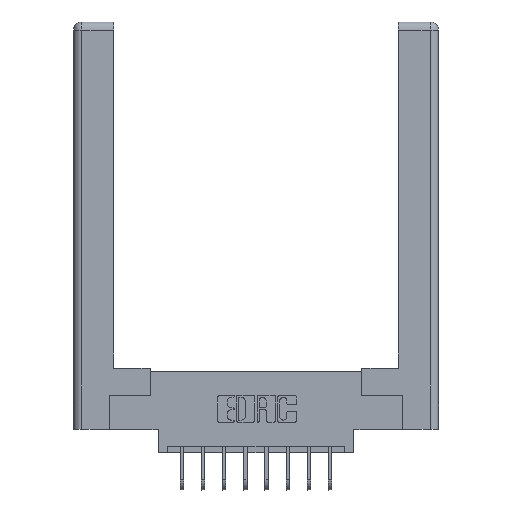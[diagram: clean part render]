
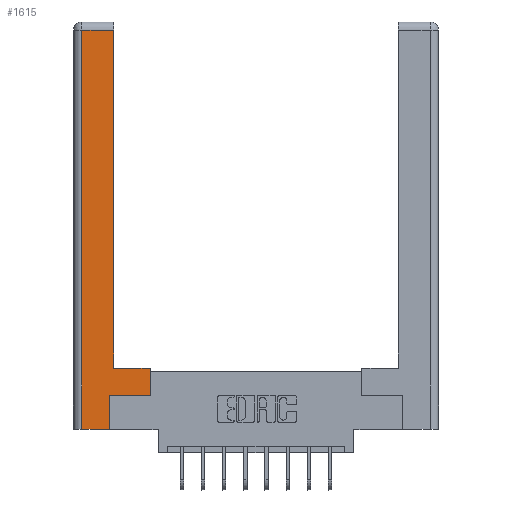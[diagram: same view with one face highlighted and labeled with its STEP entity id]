
A CAD part, top view. The second image highlights one B-rep face of the part: STEP entity #1615.
In plain terms, the highlighted planar face has unit normal (0, 0, 1).
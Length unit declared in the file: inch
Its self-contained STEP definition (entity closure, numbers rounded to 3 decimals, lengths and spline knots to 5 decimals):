
#156 = CARTESIAN_POINT ( 'NONE',  ( 0.265, 0.245, 0. ) ) ;
#361 = ORIENTED_EDGE ( 'NONE', *, *, #6981, .T. ) ;
#690 = CARTESIAN_POINT ( 'NONE',  ( 0.0615, 0., 0. ) ) ;
#691 = CARTESIAN_POINT ( 'NONE',  ( 0.565, 0.245, 0. ) ) ;
#766 = VECTOR ( 'NONE', #13962, 39.37008 ) ;
#854 = ORIENTED_EDGE ( 'NONE', *, *, #11714, .T. ) ;
#1370 = ORIENTED_EDGE ( 'NONE', *, *, #6584, .T. ) ;
#1501 = EDGE_CURVE ( 'NONE', #4162, #12065, #8631, .T. ) ;
#1615 = ADVANCED_FACE ( 'NONE', ( #4391 ), #9600, .F. ) ;
#1638 = VECTOR ( 'NONE', #10856, 39.37008 ) ;
#1649 = VECTOR ( 'NONE', #15169, 39.37008 ) ;
#2095 = VERTEX_POINT ( 'NONE', #2620 ) ;
#2319 = EDGE_CURVE ( 'NONE', #12065, #2095, #7311, .T. ) ;
#2481 = CARTESIAN_POINT ( 'NONE',  ( 0., 0., 0. ) ) ;
#2620 = CARTESIAN_POINT ( 'NONE',  ( 0.295, 0.45, 0. ) ) ;
#2752 = EDGE_CURVE ( 'NONE', #12931, #4162, #7843, .T. ) ;
#3084 = DIRECTION ( 'NONE',  ( 0., 1., 0. ) ) ;
#3595 = DIRECTION ( 'NONE',  ( 0., -1., 0. ) ) ;
#3642 = DIRECTION ( 'NONE',  ( 0., 0., -1. ) ) ;
#3760 = LINE ( 'NONE', #7287, #11484 ) ;
#3936 = AXIS2_PLACEMENT_3D ( 'NONE', #2481, #3642, #4826 ) ;
#4162 = VERTEX_POINT ( 'NONE', #691 ) ;
#4369 = CARTESIAN_POINT ( 'NONE',  ( 0.265, 0., 0. ) ) ;
#4391 = FACE_OUTER_BOUND ( 'NONE', #10382, .T. ) ;
#4430 = LINE ( 'NONE', #11430, #14558 ) ;
#4826 = DIRECTION ( 'NONE',  ( -1., 0., 0. ) ) ;
#4856 = EDGE_CURVE ( 'NONE', #7955, #14331, #3760, .T. ) ;
#5141 = ORIENTED_EDGE ( 'NONE', *, *, #1501, .T. ) ;
#5241 = DIRECTION ( 'NONE',  ( -1., 0., 0. ) ) ;
#5264 = VECTOR ( 'NONE', #7913, 39.37008 ) ;
#5302 = VERTEX_POINT ( 'NONE', #4369 ) ;
#5493 = CARTESIAN_POINT ( 'NONE',  ( 0.265, 0.245, 0. ) ) ;
#5680 = CARTESIAN_POINT ( 'NONE',  ( 0.295, 3., 0. ) ) ;
#5685 = LINE ( 'NONE', #5680, #766 ) ;
#5876 = EDGE_CURVE ( 'NONE', #5302, #12931, #7757, .T. ) ;
#6104 = ORIENTED_EDGE ( 'NONE', *, *, #2752, .T. ) ;
#6584 = EDGE_CURVE ( 'NONE', #14049, #7955, #7743, .T. ) ;
#6746 = CARTESIAN_POINT ( 'NONE',  ( 0.565, 0.245, 0. ) ) ;
#6981 = EDGE_CURVE ( 'NONE', #2095, #14049, #5685, .T. ) ;
#7035 = VECTOR ( 'NONE', #3084, 39.37008 ) ;
#7287 = CARTESIAN_POINT ( 'NONE',  ( 0.0615, 0., 0. ) ) ;
#7311 = LINE ( 'NONE', #11934, #1638 ) ;
#7551 = VECTOR ( 'NONE', #5241, 39.37008 ) ;
#7743 = LINE ( 'NONE', #13588, #7551 ) ;
#7757 = LINE ( 'NONE', #156, #7035 ) ;
#7843 = LINE ( 'NONE', #6746, #5264 ) ;
#7913 = DIRECTION ( 'NONE',  ( 1., 0., 0. ) ) ;
#7955 = VERTEX_POINT ( 'NONE', #13560 ) ;
#8631 = LINE ( 'NONE', #13912, #1649 ) ;
#8905 = CARTESIAN_POINT ( 'NONE',  ( 0.565, 0.45, 0. ) ) ;
#9097 = ORIENTED_EDGE ( 'NONE', *, *, #5876, .T. ) ;
#9600 = PLANE ( 'NONE',  #3936 ) ;
#10382 = EDGE_LOOP ( 'NONE', ( #361, #1370, #12322, #854, #9097, #6104, #5141, #11536 ) ) ;
#10856 = DIRECTION ( 'NONE',  ( -1., 0., 0. ) ) ;
#11373 = DIRECTION ( 'NONE',  ( 1., 0., 0. ) ) ;
#11430 = CARTESIAN_POINT ( 'NONE',  ( 0.265, 0., 0. ) ) ;
#11484 = VECTOR ( 'NONE', #3595, 39.37008 ) ;
#11536 = ORIENTED_EDGE ( 'NONE', *, *, #2319, .T. ) ;
#11714 = EDGE_CURVE ( 'NONE', #14331, #5302, #4430, .T. ) ;
#11871 = CARTESIAN_POINT ( 'NONE',  ( 0.295, 2.94, 0. ) ) ;
#11934 = CARTESIAN_POINT ( 'NONE',  ( 0.295, 0.45, 0. ) ) ;
#12065 = VERTEX_POINT ( 'NONE', #8905 ) ;
#12322 = ORIENTED_EDGE ( 'NONE', *, *, #4856, .T. ) ;
#12931 = VERTEX_POINT ( 'NONE', #5493 ) ;
#13560 = CARTESIAN_POINT ( 'NONE',  ( 0.0615, 2.94, 0. ) ) ;
#13588 = CARTESIAN_POINT ( 'NONE',  ( 0.0615, 2.94, 0. ) ) ;
#13912 = CARTESIAN_POINT ( 'NONE',  ( 0.565, 0.45, 0. ) ) ;
#13962 = DIRECTION ( 'NONE',  ( 0., 1., 0. ) ) ;
#14049 = VERTEX_POINT ( 'NONE', #11871 ) ;
#14331 = VERTEX_POINT ( 'NONE', #690 ) ;
#14558 = VECTOR ( 'NONE', #11373, 39.37008 ) ;
#15169 = DIRECTION ( 'NONE',  ( 0., 1., 0. ) ) ;
